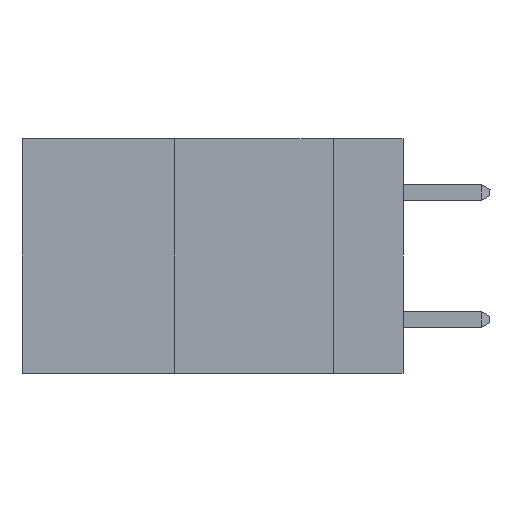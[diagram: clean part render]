
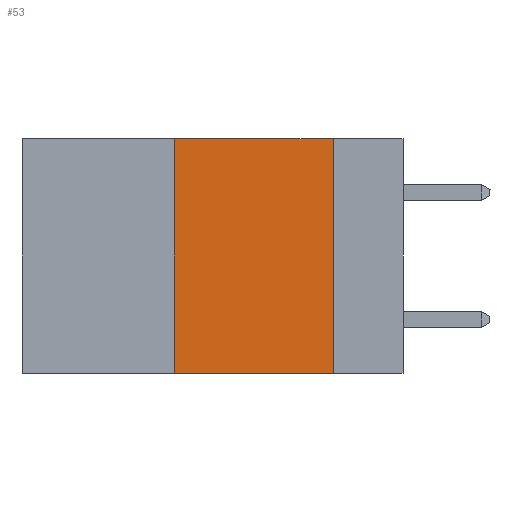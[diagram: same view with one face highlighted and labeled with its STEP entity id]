
A CAD part, left-side view. The second image highlights one B-rep face of the part: STEP entity #53.
In plain terms, the highlighted planar face has unit normal (-1, 0, 0).
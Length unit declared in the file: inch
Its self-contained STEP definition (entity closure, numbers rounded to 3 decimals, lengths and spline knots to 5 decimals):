
#41 = ORIENTED_EDGE ( 'NONE', *, *, #7051, .F. ) ;
#53 = ADVANCED_FACE ( 'NONE', ( #10975 ), #6160, .F. ) ;
#403 = EDGE_LOOP ( 'NONE', ( #41, #1494, #7682, #10430 ) ) ;
#1494 = ORIENTED_EDGE ( 'NONE', *, *, #13971, .F. ) ;
#1550 = LINE ( 'NONE', #5541, #4055 ) ;
#1895 = EDGE_CURVE ( 'NONE', #14271, #10233, #12519, .T. ) ;
#2321 = LINE ( 'NONE', #11411, #13415 ) ;
#2563 = VECTOR ( 'NONE', #11539, 39.37008 ) ;
#2717 = DIRECTION ( 'NONE',  ( 1., 0., 0. ) ) ;
#3300 = DIRECTION ( 'NONE',  ( 0., 0., -1. ) ) ;
#3725 = CARTESIAN_POINT ( 'NONE',  ( 0., 0.11, -0.37 ) ) ;
#4055 = VECTOR ( 'NONE', #13351, 39.37008 ) ;
#5101 = VERTEX_POINT ( 'NONE', #5598 ) ;
#5541 = CARTESIAN_POINT ( 'NONE',  ( 0., 0.36, 0. ) ) ;
#5598 = CARTESIAN_POINT ( 'NONE',  ( 0., 0.11, 0. ) ) ;
#5805 = LINE ( 'NONE', #10482, #2563 ) ;
#6002 = EDGE_CURVE ( 'NONE', #14271, #14138, #1550, .T. ) ;
#6160 = PLANE ( 'NONE',  #8530 ) ;
#6682 = DIRECTION ( 'NONE',  ( 0., 0., -1. ) ) ;
#7051 = EDGE_CURVE ( 'NONE', #5101, #10233, #2321, .T. ) ;
#7682 = ORIENTED_EDGE ( 'NONE', *, *, #6002, .F. ) ;
#8464 = DIRECTION ( 'NONE',  ( 0., -1., 0. ) ) ;
#8530 = AXIS2_PLACEMENT_3D ( 'NONE', #14490, #2717, #6682 ) ;
#9681 = VECTOR ( 'NONE', #8464, 39.37008 ) ;
#10233 = VERTEX_POINT ( 'NONE', #3725 ) ;
#10430 = ORIENTED_EDGE ( 'NONE', *, *, #1895, .T. ) ;
#10444 = CARTESIAN_POINT ( 'NONE',  ( 0., 0.6, -0.37 ) ) ;
#10482 = CARTESIAN_POINT ( 'NONE',  ( 0., 0.6, 0. ) ) ;
#10975 = FACE_OUTER_BOUND ( 'NONE', #403, .T. ) ;
#11411 = CARTESIAN_POINT ( 'NONE',  ( 0., 0.11, 0. ) ) ;
#11539 = DIRECTION ( 'NONE',  ( 0., -1., 0. ) ) ;
#12519 = LINE ( 'NONE', #10444, #9681 ) ;
#12673 = CARTESIAN_POINT ( 'NONE',  ( 0., 0.36, 0. ) ) ;
#13351 = DIRECTION ( 'NONE',  ( 0., 0., 1. ) ) ;
#13415 = VECTOR ( 'NONE', #3300, 39.37008 ) ;
#13971 = EDGE_CURVE ( 'NONE', #14138, #5101, #5805, .T. ) ;
#14138 = VERTEX_POINT ( 'NONE', #12673 ) ;
#14271 = VERTEX_POINT ( 'NONE', #14819 ) ;
#14490 = CARTESIAN_POINT ( 'NONE',  ( 0., 0.6, 0. ) ) ;
#14819 = CARTESIAN_POINT ( 'NONE',  ( 0., 0.36, -0.37 ) ) ;
